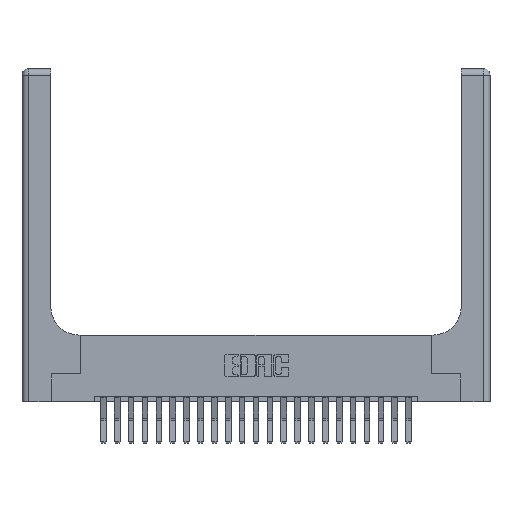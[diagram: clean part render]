
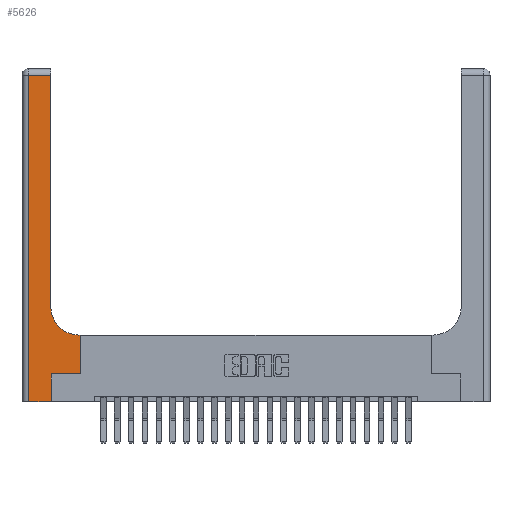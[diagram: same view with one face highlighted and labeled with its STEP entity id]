
A CAD part, top view. The second image highlights one B-rep face of the part: STEP entity #5626.
In plain terms, the highlighted planar face has unit normal (0, 0, 1).
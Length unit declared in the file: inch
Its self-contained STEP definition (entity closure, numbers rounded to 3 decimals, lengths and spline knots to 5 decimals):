
#184 = AXIS2_PLACEMENT_3D ( 'NONE', #10517, #19138, #20947 ) ;
#741 = LINE ( 'NONE', #11893, #2117 ) ;
#932 = EDGE_CURVE ( 'NONE', #14975, #22330, #5210, .T. ) ;
#1169 = CARTESIAN_POINT ( 'NONE',  ( 0.26, 0.6, 0.37 ) ) ;
#1251 = VECTOR ( 'NONE', #9696, 39.37008 ) ;
#1281 = CARTESIAN_POINT ( 'NONE',  ( 0.265, 0.25, 0.37 ) ) ;
#1619 = VECTOR ( 'NONE', #7123, 39.37008 ) ;
#2013 = AXIS2_PLACEMENT_3D ( 'NONE', #7912, #18363, #20216 ) ;
#2117 = VECTOR ( 'NONE', #3091, 39.37008 ) ;
#2213 = EDGE_CURVE ( 'NONE', #16644, #9521, #741, .T. ) ;
#2500 = PLANE ( 'NONE',  #2013 ) ;
#2709 = ORIENTED_EDGE ( 'NONE', *, *, #932, .T. ) ;
#2782 = DIRECTION ( 'NONE',  ( -1., 0., 0. ) ) ;
#3091 = DIRECTION ( 'NONE',  ( 0., -1., 0. ) ) ;
#3130 = ORIENTED_EDGE ( 'NONE', *, *, #15989, .T. ) ;
#5210 = CIRCLE ( 'NONE', #184, 0.25 ) ;
#5389 = LINE ( 'NONE', #14844, #7891 ) ;
#5520 = VERTEX_POINT ( 'NONE', #14752 ) ;
#5626 = ADVANCED_FACE ( 'NONE', ( #20733 ), #2500, .F. ) ;
#7082 = LINE ( 'NONE', #1169, #19748 ) ;
#7123 = DIRECTION ( 'NONE',  ( 1., 0., 0. ) ) ;
#7359 = LINE ( 'NONE', #18558, #22546 ) ;
#7891 = VECTOR ( 'NONE', #9556, 39.37008 ) ;
#7912 = CARTESIAN_POINT ( 'NONE',  ( 0., 3., 0.37 ) ) ;
#8689 = CARTESIAN_POINT ( 'NONE',  ( 0.265, 0., 0.37 ) ) ;
#9022 = EDGE_CURVE ( 'NONE', #5520, #15559, #9705, .T. ) ;
#9521 = VERTEX_POINT ( 'NONE', #15676 ) ;
#9556 = DIRECTION ( 'NONE',  ( -1., 0., 0. ) ) ;
#9581 = VERTEX_POINT ( 'NONE', #8689 ) ;
#9621 = CARTESIAN_POINT ( 'NONE',  ( 0.26, 3., 0.37 ) ) ;
#9696 = DIRECTION ( 'NONE',  ( 0., 1., 0. ) ) ;
#9705 = LINE ( 'NONE', #1281, #15742 ) ;
#10362 = CARTESIAN_POINT ( 'NONE',  ( 0.528, 0.25, 0.37 ) ) ;
#10433 = EDGE_CURVE ( 'NONE', #9521, #9581, #20095, .T. ) ;
#10517 = CARTESIAN_POINT ( 'NONE',  ( 0.51, 0.85, 0.37 ) ) ;
#10618 = ORIENTED_EDGE ( 'NONE', *, *, #12744, .T. ) ;
#11577 = DIRECTION ( 'NONE',  ( 0., 1., 0. ) ) ;
#11810 = EDGE_CURVE ( 'NONE', #9581, #5520, #7359, .T. ) ;
#11893 = CARTESIAN_POINT ( 'NONE',  ( 0.06, 3., 0.37 ) ) ;
#12159 = ORIENTED_EDGE ( 'NONE', *, *, #10433, .T. ) ;
#12302 = ORIENTED_EDGE ( 'NONE', *, *, #9022, .T. ) ;
#12411 = EDGE_CURVE ( 'NONE', #16383, #16644, #5389, .T. ) ;
#12744 = EDGE_CURVE ( 'NONE', #22330, #16383, #16967, .T. ) ;
#14187 = VERTEX_POINT ( 'NONE', #17843 ) ;
#14470 = CARTESIAN_POINT ( 'NONE',  ( 0.26, 0.85, 0.37 ) ) ;
#14752 = CARTESIAN_POINT ( 'NONE',  ( 0.265, 0.25, 0.37 ) ) ;
#14844 = CARTESIAN_POINT ( 'NONE',  ( 0., 2.94, 0.37 ) ) ;
#14975 = VERTEX_POINT ( 'NONE', #15273 ) ;
#15163 = CARTESIAN_POINT ( 'NONE',  ( 0.528, 0.25, 0.37 ) ) ;
#15268 = ORIENTED_EDGE ( 'NONE', *, *, #12411, .T. ) ;
#15273 = CARTESIAN_POINT ( 'NONE',  ( 0.51, 0.6, 0.37 ) ) ;
#15559 = VERTEX_POINT ( 'NONE', #15163 ) ;
#15676 = CARTESIAN_POINT ( 'NONE',  ( 0.06, 0., 0.37 ) ) ;
#15742 = VECTOR ( 'NONE', #16925, 39.37008 ) ;
#15989 = EDGE_CURVE ( 'NONE', #14187, #14975, #7082, .T. ) ;
#16321 = ORIENTED_EDGE ( 'NONE', *, *, #2213, .T. ) ;
#16383 = VERTEX_POINT ( 'NONE', #16452 ) ;
#16452 = CARTESIAN_POINT ( 'NONE',  ( 0.26, 2.94, 0.37 ) ) ;
#16644 = VERTEX_POINT ( 'NONE', #20447 ) ;
#16807 = VECTOR ( 'NONE', #19051, 39.37008 ) ;
#16925 = DIRECTION ( 'NONE',  ( 1., 0., 0. ) ) ;
#16967 = LINE ( 'NONE', #9621, #1251 ) ;
#17127 = ORIENTED_EDGE ( 'NONE', *, *, #11810, .T. ) ;
#17669 = CARTESIAN_POINT ( 'NONE',  ( 0., 0., 0.37 ) ) ;
#17843 = CARTESIAN_POINT ( 'NONE',  ( 0.528, 0.6, 0.37 ) ) ;
#18363 = DIRECTION ( 'NONE',  ( 0., 0., -1. ) ) ;
#18525 = EDGE_LOOP ( 'NONE', ( #10618, #15268, #16321, #12159, #17127, #12302, #21173, #3130, #2709 ) ) ;
#18558 = CARTESIAN_POINT ( 'NONE',  ( 0.265, 0., 0.37 ) ) ;
#19051 = DIRECTION ( 'NONE',  ( 0., 1., 0. ) ) ;
#19138 = DIRECTION ( 'NONE',  ( 0., 0., -1. ) ) ;
#19277 = LINE ( 'NONE', #10362, #16807 ) ;
#19748 = VECTOR ( 'NONE', #2782, 39.37008 ) ;
#20044 = EDGE_CURVE ( 'NONE', #15559, #14187, #19277, .T. ) ;
#20095 = LINE ( 'NONE', #17669, #1619 ) ;
#20216 = DIRECTION ( 'NONE',  ( -1., 0., 0. ) ) ;
#20447 = CARTESIAN_POINT ( 'NONE',  ( 0.06, 2.94, 0.37 ) ) ;
#20733 = FACE_OUTER_BOUND ( 'NONE', #18525, .T. ) ;
#20947 = DIRECTION ( 'NONE',  ( 1., 0., 0. ) ) ;
#21173 = ORIENTED_EDGE ( 'NONE', *, *, #20044, .T. ) ;
#22330 = VERTEX_POINT ( 'NONE', #14470 ) ;
#22546 = VECTOR ( 'NONE', #11577, 39.37008 ) ;
